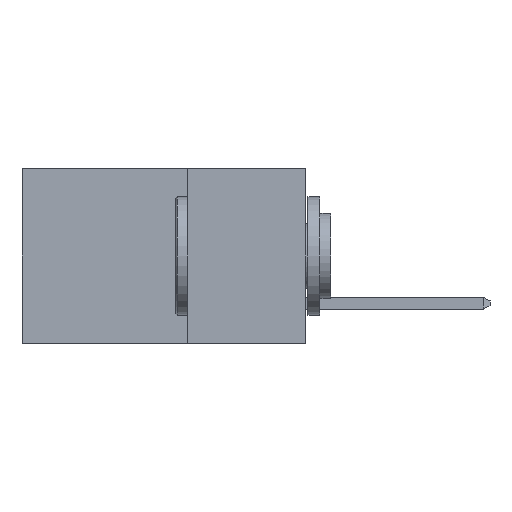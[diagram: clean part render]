
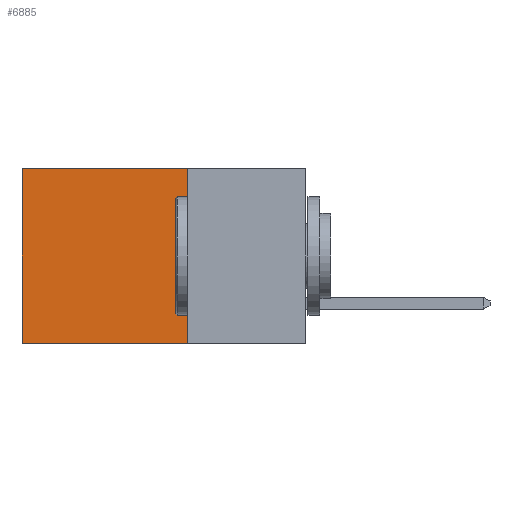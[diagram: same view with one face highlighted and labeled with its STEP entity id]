
A CAD part, left-side view. The second image highlights one B-rep face of the part: STEP entity #6885.
In plain terms, the highlighted planar face has unit normal (-1, 0, 0).
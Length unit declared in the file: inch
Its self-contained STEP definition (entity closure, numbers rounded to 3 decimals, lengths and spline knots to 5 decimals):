
#683 = DIRECTION ( 'NONE',  ( 0., 0., -1. ) ) ;
#840 = ORIENTED_EDGE ( 'NONE', *, *, #4731, .F. ) ;
#1232 = EDGE_LOOP ( 'NONE', ( #4417, #840, #6226, #10756 ) ) ;
#1348 = VECTOR ( 'NONE', #683, 39.37008 ) ;
#1551 = VECTOR ( 'NONE', #10746, 39.37008 ) ;
#1866 = CARTESIAN_POINT ( 'NONE',  ( 0.298, 0.25, 0. ) ) ;
#2013 = LINE ( 'NONE', #9572, #6266 ) ;
#2277 = PLANE ( 'NONE',  #6602 ) ;
#3153 = DIRECTION ( 'NONE',  ( 0., 0., -1. ) ) ;
#3455 = CARTESIAN_POINT ( 'NONE',  ( 0.298, 0.6, -0.37 ) ) ;
#3673 = CARTESIAN_POINT ( 'NONE',  ( 0.298, 0.6, 0. ) ) ;
#3686 = LINE ( 'NONE', #9972, #1348 ) ;
#3879 = LINE ( 'NONE', #8969, #1551 ) ;
#4043 = VERTEX_POINT ( 'NONE', #3673 ) ;
#4417 = ORIENTED_EDGE ( 'NONE', *, *, #6520, .T. ) ;
#4731 = EDGE_CURVE ( 'NONE', #6952, #7116, #9450, .T. ) ;
#5757 = CARTESIAN_POINT ( 'NONE',  ( 0.298, 0.25, -0.37 ) ) ;
#6226 = ORIENTED_EDGE ( 'NONE', *, *, #9878, .F. ) ;
#6266 = VECTOR ( 'NONE', #9610, 39.37008 ) ;
#6421 = VERTEX_POINT ( 'NONE', #1866 ) ;
#6520 = EDGE_CURVE ( 'NONE', #4043, #7116, #2013, .T. ) ;
#6602 = AXIS2_PLACEMENT_3D ( 'NONE', #8995, #8179, #3153 ) ;
#6885 = ADVANCED_FACE ( 'NONE', ( #10111 ), #2277, .F. ) ;
#6935 = VECTOR ( 'NONE', #7924, 39.37008 ) ;
#6952 = VERTEX_POINT ( 'NONE', #5757 ) ;
#7116 = VERTEX_POINT ( 'NONE', #3455 ) ;
#7924 = DIRECTION ( 'NONE',  ( 0., 1., 0. ) ) ;
#8089 = EDGE_CURVE ( 'NONE', #6421, #4043, #3879, .T. ) ;
#8179 = DIRECTION ( 'NONE',  ( 1., 0., 0. ) ) ;
#8969 = CARTESIAN_POINT ( 'NONE',  ( 0.298, 0.25, 0. ) ) ;
#8995 = CARTESIAN_POINT ( 'NONE',  ( 0.298, 0.25, 0. ) ) ;
#9450 = LINE ( 'NONE', #10520, #6935 ) ;
#9572 = CARTESIAN_POINT ( 'NONE',  ( 0.298, 0.6, 0. ) ) ;
#9610 = DIRECTION ( 'NONE',  ( 0., 0., -1. ) ) ;
#9878 = EDGE_CURVE ( 'NONE', #6421, #6952, #3686, .T. ) ;
#9972 = CARTESIAN_POINT ( 'NONE',  ( 0.298, 0.25, 0. ) ) ;
#10111 = FACE_OUTER_BOUND ( 'NONE', #1232, .T. ) ;
#10520 = CARTESIAN_POINT ( 'NONE',  ( 0.298, 0.25, -0.37 ) ) ;
#10746 = DIRECTION ( 'NONE',  ( 0., 1., 0. ) ) ;
#10756 = ORIENTED_EDGE ( 'NONE', *, *, #8089, .T. ) ;
